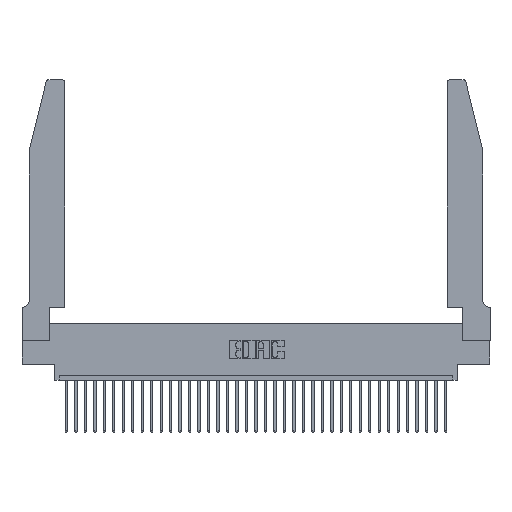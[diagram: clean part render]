
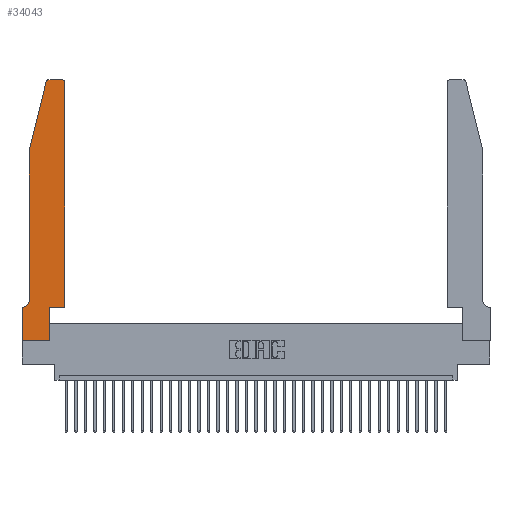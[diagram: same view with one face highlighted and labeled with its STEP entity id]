
A CAD part, top view. The second image highlights one B-rep face of the part: STEP entity #34043.
In plain terms, the highlighted planar face has unit normal (0, 0, 1).
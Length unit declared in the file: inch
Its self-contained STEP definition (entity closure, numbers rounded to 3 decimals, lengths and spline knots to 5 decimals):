
#195 = CARTESIAN_POINT ( 'NONE',  ( 0.4505, 0.35, 0.37 ) ) ;
#1132 = CIRCLE ( 'NONE', #1358, 0.03 ) ;
#1358 = AXIS2_PLACEMENT_3D ( 'NONE', #33334, #27869, #25189 ) ;
#1367 = CARTESIAN_POINT ( 'NONE',  ( 0.0755, 2., 0.37 ) ) ;
#1517 = CARTESIAN_POINT ( 'NONE',  ( 0.25487, 2.72718, 0.37 ) ) ;
#2158 = EDGE_CURVE ( 'NONE', #19403, #33115, #24525, .T. ) ;
#2697 = ORIENTED_EDGE ( 'NONE', *, *, #20431, .T. ) ;
#3071 = AXIS2_PLACEMENT_3D ( 'NONE', #35824, #30497, #11125 ) ;
#3137 = EDGE_CURVE ( 'NONE', #16295, #19987, #1132, .T. ) ;
#4253 = VECTOR ( 'NONE', #15012, 39.37008 ) ;
#4358 = CARTESIAN_POINT ( 'NONE',  ( 0.2865, 0., 0.37 ) ) ;
#4954 = VECTOR ( 'NONE', #5573, 39.37008 ) ;
#5573 = DIRECTION ( 'NONE',  ( -1., 0., 0. ) ) ;
#7400 = EDGE_CURVE ( 'NONE', #33115, #35688, #9069, .T. ) ;
#7554 = ORIENTED_EDGE ( 'NONE', *, *, #3137, .T. ) ;
#7875 = EDGE_CURVE ( 'NONE', #10973, #16244, #32914, .T. ) ;
#9069 = CIRCLE ( 'NONE', #3071, 0.07 ) ;
#9274 = ORIENTED_EDGE ( 'NONE', *, *, #14702, .T. ) ;
#9341 = LINE ( 'NONE', #34172, #23665 ) ;
#9727 = DIRECTION ( 'NONE',  ( 0., -1., 0. ) ) ;
#10033 = VERTEX_POINT ( 'NONE', #195 ) ;
#10350 = VECTOR ( 'NONE', #28202, 39.37008 ) ;
#10351 = CARTESIAN_POINT ( 'NONE',  ( 0.0755, 2., 0.37 ) ) ;
#10403 = ORIENTED_EDGE ( 'NONE', *, *, #13516, .T. ) ;
#10973 = VERTEX_POINT ( 'NONE', #11593 ) ;
#11125 = DIRECTION ( 'NONE',  ( -1., 0., 0. ) ) ;
#11514 = CARTESIAN_POINT ( 'NONE',  ( 0., 0., 0.37 ) ) ;
#11593 = CARTESIAN_POINT ( 'NONE',  ( 0., 0., 0.37 ) ) ;
#11618 = ORIENTED_EDGE ( 'NONE', *, *, #26617, .T. ) ;
#11639 = LINE ( 'NONE', #17062, #4253 ) ;
#12314 = DIRECTION ( 'NONE',  ( 1., 0., 0. ) ) ;
#12405 = VECTOR ( 'NONE', #9727, 39.37008 ) ;
#13436 = CARTESIAN_POINT ( 'NONE',  ( 0.0755, 0.35, 0.37 ) ) ;
#13462 = LINE ( 'NONE', #26730, #23023 ) ;
#13516 = EDGE_CURVE ( 'NONE', #35688, #26553, #31064, .T. ) ;
#13654 = LINE ( 'NONE', #27839, #4954 ) ;
#13821 = VERTEX_POINT ( 'NONE', #14404 ) ;
#14004 = EDGE_LOOP ( 'NONE', ( #9274, #7554, #21011, #20402, #28717, #10403, #23860, #16920, #14468, #2697, #26873, #11618 ) ) ;
#14404 = CARTESIAN_POINT ( 'NONE',  ( 0.4505, 2.72, 0.37 ) ) ;
#14468 = ORIENTED_EDGE ( 'NONE', *, *, #25978, .T. ) ;
#14702 = EDGE_CURVE ( 'NONE', #22218, #16295, #13654, .T. ) ;
#15012 = DIRECTION ( 'NONE',  ( 0., -1., 0. ) ) ;
#15474 = VECTOR ( 'NONE', #35353, 39.37008 ) ;
#16244 = VERTEX_POINT ( 'NONE', #4358 ) ;
#16295 = VERTEX_POINT ( 'NONE', #27844 ) ;
#16458 = AXIS2_PLACEMENT_3D ( 'NONE', #18368, #34813, #20797 ) ;
#16920 = ORIENTED_EDGE ( 'NONE', *, *, #7875, .T. ) ;
#17062 = CARTESIAN_POINT ( 'NONE',  ( 0., 0., 0.37 ) ) ;
#18368 = CARTESIAN_POINT ( 'NONE',  ( 0.4205, 2.72, 0.37 ) ) ;
#18375 = DIRECTION ( 'NONE',  ( -0.239, -0.971, 0. ) ) ;
#19403 = VERTEX_POINT ( 'NONE', #31161 ) ;
#19987 = VERTEX_POINT ( 'NONE', #1517 ) ;
#20402 = ORIENTED_EDGE ( 'NONE', *, *, #2158, .T. ) ;
#20431 = EDGE_CURVE ( 'NONE', #20607, #10033, #13462, .T. ) ;
#20607 = VERTEX_POINT ( 'NONE', #29997 ) ;
#20797 = DIRECTION ( 'NONE',  ( 1., 0., 0. ) ) ;
#20880 = VECTOR ( 'NONE', #18375, 39.37008 ) ;
#21011 = ORIENTED_EDGE ( 'NONE', *, *, #34266, .T. ) ;
#21534 = AXIS2_PLACEMENT_3D ( 'NONE', #26441, #28773, #12314 ) ;
#21661 = CARTESIAN_POINT ( 'NONE',  ( 0.4205, 2.75, 0.37 ) ) ;
#21740 = LINE ( 'NONE', #10351, #20880 ) ;
#21985 = EDGE_CURVE ( 'NONE', #26553, #10973, #11639, .T. ) ;
#22218 = VERTEX_POINT ( 'NONE', #21661 ) ;
#23023 = VECTOR ( 'NONE', #29781, 39.37008 ) ;
#23665 = VECTOR ( 'NONE', #34410, 39.37008 ) ;
#23860 = ORIENTED_EDGE ( 'NONE', *, *, #21985, .T. ) ;
#24525 = LINE ( 'NONE', #1367, #12405 ) ;
#25189 = DIRECTION ( 'NONE',  ( 1., 0., 0. ) ) ;
#25577 = CARTESIAN_POINT ( 'NONE',  ( 0.0055, 0.35, 0.37 ) ) ;
#25978 = EDGE_CURVE ( 'NONE', #16244, #20607, #27651, .T. ) ;
#26427 = CARTESIAN_POINT ( 'NONE',  ( 0.2865, 0.35, 0.37 ) ) ;
#26441 = CARTESIAN_POINT ( 'NONE',  ( 0., 0.35, 0.37 ) ) ;
#26553 = VERTEX_POINT ( 'NONE', #32038 ) ;
#26617 = EDGE_CURVE ( 'NONE', #13821, #22218, #28033, .T. ) ;
#26730 = CARTESIAN_POINT ( 'NONE',  ( 0.4505, 0.35, 0.37 ) ) ;
#26873 = ORIENTED_EDGE ( 'NONE', *, *, #27185, .T. ) ;
#27185 = EDGE_CURVE ( 'NONE', #10033, #13821, #9341, .T. ) ;
#27651 = LINE ( 'NONE', #26427, #33264 ) ;
#27839 = CARTESIAN_POINT ( 'NONE',  ( 0.2605, 2.75, 0.37 ) ) ;
#27844 = CARTESIAN_POINT ( 'NONE',  ( 0.284, 2.75, 0.37 ) ) ;
#27869 = DIRECTION ( 'NONE',  ( 0., 0., 1. ) ) ;
#28033 = CIRCLE ( 'NONE', #16458, 0.03 ) ;
#28202 = DIRECTION ( 'NONE',  ( 1., 0., 0. ) ) ;
#28717 = ORIENTED_EDGE ( 'NONE', *, *, #7400, .T. ) ;
#28773 = DIRECTION ( 'NONE',  ( 0., 0., 1. ) ) ;
#29781 = DIRECTION ( 'NONE',  ( 1., 0., 0. ) ) ;
#29997 = CARTESIAN_POINT ( 'NONE',  ( 0.2865, 0.35, 0.37 ) ) ;
#30497 = DIRECTION ( 'NONE',  ( 0., 0., -1. ) ) ;
#31064 = LINE ( 'NONE', #13436, #15474 ) ;
#31161 = CARTESIAN_POINT ( 'NONE',  ( 0.0755, 2., 0.37 ) ) ;
#32026 = DIRECTION ( 'NONE',  ( 0., 1., 0. ) ) ;
#32038 = CARTESIAN_POINT ( 'NONE',  ( 0., 0.35, 0.37 ) ) ;
#32914 = LINE ( 'NONE', #11514, #10350 ) ;
#33115 = VERTEX_POINT ( 'NONE', #35142 ) ;
#33264 = VECTOR ( 'NONE', #32026, 39.37008 ) ;
#33334 = CARTESIAN_POINT ( 'NONE',  ( 0.284, 2.72, 0.37 ) ) ;
#34043 = ADVANCED_FACE ( 'NONE', ( #34708 ), #34334, .T. ) ;
#34172 = CARTESIAN_POINT ( 'NONE',  ( 0.4505, 0.35, 0.37 ) ) ;
#34266 = EDGE_CURVE ( 'NONE', #19987, #19403, #21740, .T. ) ;
#34334 = PLANE ( 'NONE',  #21534 ) ;
#34410 = DIRECTION ( 'NONE',  ( 0., 1., 0. ) ) ;
#34708 = FACE_OUTER_BOUND ( 'NONE', #14004, .T. ) ;
#34813 = DIRECTION ( 'NONE',  ( 0., 0., 1. ) ) ;
#35142 = CARTESIAN_POINT ( 'NONE',  ( 0.0755, 0.42, 0.37 ) ) ;
#35353 = DIRECTION ( 'NONE',  ( -1., 0., 0. ) ) ;
#35688 = VERTEX_POINT ( 'NONE', #25577 ) ;
#35824 = CARTESIAN_POINT ( 'NONE',  ( 0.0055, 0.42, 0.37 ) ) ;
